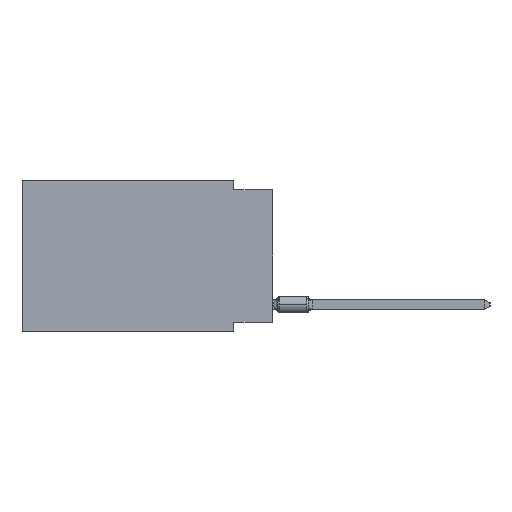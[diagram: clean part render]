
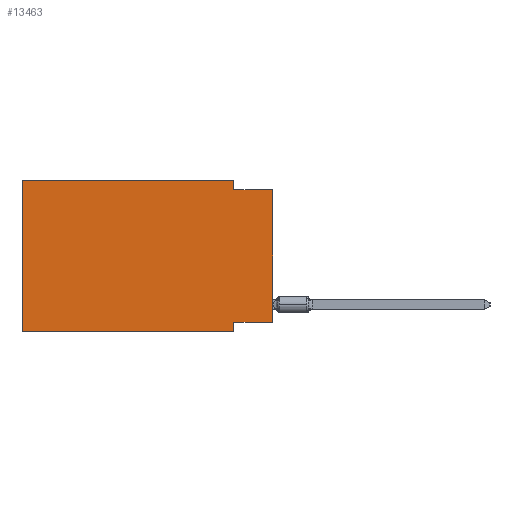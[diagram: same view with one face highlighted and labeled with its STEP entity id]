
A CAD part, left-side view. The second image highlights one B-rep face of the part: STEP entity #13463.
In plain terms, the highlighted planar face has unit normal (-1, 0, 0).
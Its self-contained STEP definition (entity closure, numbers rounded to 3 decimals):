
#2 = VERTEX_POINT ( 'NONE', #16035 ) ;
#76 = FACE_OUTER_BOUND ( 'NONE', #3063, .T. ) ;
#1212 = VECTOR ( 'NONE', #2964, 1000. ) ;
#1306 = LINE ( 'NONE', #23031, #29418 ) ;
#2285 = EDGE_CURVE ( 'NONE', #16790, #6437, #35531, .T. ) ;
#2964 = DIRECTION ( 'NONE',  ( 0., 1., 0. ) ) ;
#3063 = EDGE_LOOP ( 'NONE', ( #17503, #23572, #19662, #7987, #15601, #17096, #10431, #13228 ) ) ;
#3131 = DIRECTION ( 'NONE',  ( 0., 0., -1. ) ) ;
#3558 = LINE ( 'NONE', #28521, #32374 ) ;
#5015 = EDGE_CURVE ( 'NONE', #39123, #2, #24074, .T. ) ;
#5714 = DIRECTION ( 'NONE',  ( 0., 0., -1. ) ) ;
#6437 = VERTEX_POINT ( 'NONE', #9860 ) ;
#6997 = DIRECTION ( 'NONE',  ( 0., -1., 0. ) ) ;
#7987 = ORIENTED_EDGE ( 'NONE', *, *, #33246, .F. ) ;
#8887 = EDGE_CURVE ( 'NONE', #38525, #34899, #24685, .T. ) ;
#9860 = CARTESIAN_POINT ( 'NONE',  ( 0., 2.54, -9.906 ) ) ;
#10431 = ORIENTED_EDGE ( 'NONE', *, *, #22056, .F. ) ;
#10835 = AXIS2_PLACEMENT_3D ( 'NONE', #28693, #25443, #3131 ) ;
#11134 = CARTESIAN_POINT ( 'NONE',  ( 0., 2.54, 0. ) ) ;
#11822 = EDGE_CURVE ( 'NONE', #16790, #29456, #29984, .T. ) ;
#12300 = DIRECTION ( 'NONE',  ( 0., 0., -1. ) ) ;
#13228 = ORIENTED_EDGE ( 'NONE', *, *, #5015, .F. ) ;
#13431 = VERTEX_POINT ( 'NONE', #27907 ) ;
#13463 = ADVANCED_FACE ( 'NONE', ( #76 ), #37277, .F. ) ;
#13676 = CARTESIAN_POINT ( 'NONE',  ( 0., 2.54, -0.635 ) ) ;
#14235 = LINE ( 'NONE', #38628, #19350 ) ;
#15601 = ORIENTED_EDGE ( 'NONE', *, *, #11822, .F. ) ;
#16035 = CARTESIAN_POINT ( 'NONE',  ( 0., 2.54, -9.271 ) ) ;
#16232 = DIRECTION ( 'NONE',  ( 0., -1., 0. ) ) ;
#16253 = EDGE_CURVE ( 'NONE', #34899, #13431, #14235, .T. ) ;
#16790 = VERTEX_POINT ( 'NONE', #40000 ) ;
#17096 = ORIENTED_EDGE ( 'NONE', *, *, #2285, .T. ) ;
#17479 = DIRECTION ( 'NONE',  ( 0., -1., 0. ) ) ;
#17503 = ORIENTED_EDGE ( 'NONE', *, *, #21769, .T. ) ;
#18289 = VECTOR ( 'NONE', #12300, 1000. ) ;
#19350 = VECTOR ( 'NONE', #17479, 1000. ) ;
#19662 = ORIENTED_EDGE ( 'NONE', *, *, #8887, .F. ) ;
#20623 = CARTESIAN_POINT ( 'NONE',  ( 0., 0., -9.271 ) ) ;
#21769 = EDGE_CURVE ( 'NONE', #39123, #13431, #1306, .T. ) ;
#22056 = EDGE_CURVE ( 'NONE', #2, #6437, #24184, .T. ) ;
#22407 = VECTOR ( 'NONE', #27135, 1000. ) ;
#23031 = CARTESIAN_POINT ( 'NONE',  ( 0., 0., 0. ) ) ;
#23572 = ORIENTED_EDGE ( 'NONE', *, *, #16253, .F. ) ;
#24074 = LINE ( 'NONE', #20623, #1212 ) ;
#24184 = LINE ( 'NONE', #26842, #29165 ) ;
#24685 = LINE ( 'NONE', #37098, #18289 ) ;
#25443 = DIRECTION ( 'NONE',  ( 1., 0., 0. ) ) ;
#25585 = CARTESIAN_POINT ( 'NONE',  ( 0., 16.383, -9.906 ) ) ;
#26299 = DIRECTION ( 'NONE',  ( 0., 0., 1. ) ) ;
#26842 = CARTESIAN_POINT ( 'NONE',  ( 0., 2.54, -9.906 ) ) ;
#27135 = DIRECTION ( 'NONE',  ( 0., 0., 1. ) ) ;
#27907 = CARTESIAN_POINT ( 'NONE',  ( 0., 0., -0.635 ) ) ;
#28521 = CARTESIAN_POINT ( 'NONE',  ( 0., 16.383, 0. ) ) ;
#28693 = CARTESIAN_POINT ( 'NONE',  ( 0., 16.383, 0. ) ) ;
#29165 = VECTOR ( 'NONE', #5714, 1000. ) ;
#29418 = VECTOR ( 'NONE', #26299, 1000. ) ;
#29456 = VERTEX_POINT ( 'NONE', #35504 ) ;
#29984 = LINE ( 'NONE', #39334, #22407 ) ;
#30551 = CARTESIAN_POINT ( 'NONE',  ( 0., 0., -9.271 ) ) ;
#32374 = VECTOR ( 'NONE', #6997, 1000. ) ;
#33246 = EDGE_CURVE ( 'NONE', #29456, #38525, #3558, .T. ) ;
#34190 = VECTOR ( 'NONE', #16232, 1000. ) ;
#34899 = VERTEX_POINT ( 'NONE', #13676 ) ;
#35504 = CARTESIAN_POINT ( 'NONE',  ( 0., 16.383, 0. ) ) ;
#35531 = LINE ( 'NONE', #25585, #34190 ) ;
#37098 = CARTESIAN_POINT ( 'NONE',  ( 0., 2.54, 0. ) ) ;
#37277 = PLANE ( 'NONE',  #10835 ) ;
#38525 = VERTEX_POINT ( 'NONE', #11134 ) ;
#38628 = CARTESIAN_POINT ( 'NONE',  ( 0., 0., -0.635 ) ) ;
#39123 = VERTEX_POINT ( 'NONE', #30551 ) ;
#39334 = CARTESIAN_POINT ( 'NONE',  ( 0., 16.383, 0. ) ) ;
#40000 = CARTESIAN_POINT ( 'NONE',  ( 0., 16.383, -9.906 ) ) ;
